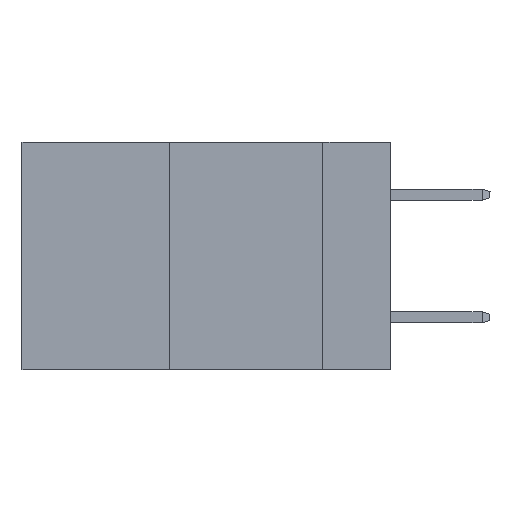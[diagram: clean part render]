
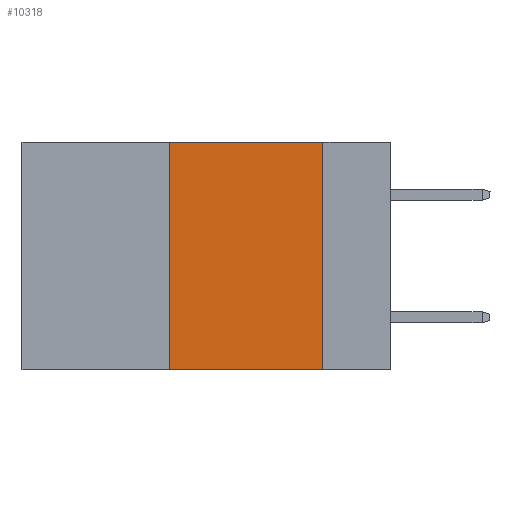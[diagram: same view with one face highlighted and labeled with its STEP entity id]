
A CAD part, left-side view. The second image highlights one B-rep face of the part: STEP entity #10318.
In plain terms, the highlighted planar face has unit normal (-1, 0, 0).
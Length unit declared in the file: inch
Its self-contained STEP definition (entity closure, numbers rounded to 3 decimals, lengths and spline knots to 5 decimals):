
#427 = CARTESIAN_POINT ( 'NONE',  ( 0., 0.11, 0. ) ) ;
#513 = CARTESIAN_POINT ( 'NONE',  ( 0., 0.36, 0. ) ) ;
#746 = EDGE_CURVE ( 'NONE', #7738, #28120, #8736, .T. ) ;
#1292 = VECTOR ( 'NONE', #10631, 39.37008 ) ;
#2387 = LINE ( 'NONE', #29016, #27207 ) ;
#4944 = VECTOR ( 'NONE', #24610, 39.37008 ) ;
#5019 = DIRECTION ( 'NONE',  ( 0., 0., -1. ) ) ;
#6196 = PLANE ( 'NONE',  #29445 ) ;
#7738 = VERTEX_POINT ( 'NONE', #27788 ) ;
#8736 = LINE ( 'NONE', #27074, #4944 ) ;
#10318 = ADVANCED_FACE ( 'NONE', ( #19518 ), #6196, .F. ) ;
#10631 = DIRECTION ( 'NONE',  ( 0., 0., 1. ) ) ;
#11008 = CARTESIAN_POINT ( 'NONE',  ( 0., 0.6, 0. ) ) ;
#14461 = ORIENTED_EDGE ( 'NONE', *, *, #14971, .F. ) ;
#14971 = EDGE_CURVE ( 'NONE', #23796, #28120, #2387, .T. ) ;
#18258 = DIRECTION ( 'NONE',  ( 0., 0., -1. ) ) ;
#19518 = FACE_OUTER_BOUND ( 'NONE', #21424, .T. ) ;
#20540 = ORIENTED_EDGE ( 'NONE', *, *, #25061, .F. ) ;
#20684 = CARTESIAN_POINT ( 'NONE',  ( 0., 0.36, 0. ) ) ;
#21006 = ORIENTED_EDGE ( 'NONE', *, *, #746, .T. ) ;
#21424 = EDGE_LOOP ( 'NONE', ( #14461, #29917, #20540, #21006 ) ) ;
#21808 = VECTOR ( 'NONE', #30907, 39.37008 ) ;
#22946 = CARTESIAN_POINT ( 'NONE',  ( 0., 0.11, -0.37 ) ) ;
#23267 = DIRECTION ( 'NONE',  ( 1., 0., 0. ) ) ;
#23796 = VERTEX_POINT ( 'NONE', #427 ) ;
#24610 = DIRECTION ( 'NONE',  ( 0., -1., 0. ) ) ;
#25061 = EDGE_CURVE ( 'NONE', #7738, #27080, #30635, .T. ) ;
#27074 = CARTESIAN_POINT ( 'NONE',  ( 0., 0.6, -0.37 ) ) ;
#27080 = VERTEX_POINT ( 'NONE', #20684 ) ;
#27207 = VECTOR ( 'NONE', #5019, 39.37008 ) ;
#27525 = LINE ( 'NONE', #28614, #21808 ) ;
#27788 = CARTESIAN_POINT ( 'NONE',  ( 0., 0.36, -0.37 ) ) ;
#28120 = VERTEX_POINT ( 'NONE', #22946 ) ;
#28614 = CARTESIAN_POINT ( 'NONE',  ( 0., 0.6, 0. ) ) ;
#28946 = EDGE_CURVE ( 'NONE', #27080, #23796, #27525, .T. ) ;
#29016 = CARTESIAN_POINT ( 'NONE',  ( 0., 0.11, 0. ) ) ;
#29445 = AXIS2_PLACEMENT_3D ( 'NONE', #11008, #23267, #18258 ) ;
#29917 = ORIENTED_EDGE ( 'NONE', *, *, #28946, .F. ) ;
#30635 = LINE ( 'NONE', #513, #1292 ) ;
#30907 = DIRECTION ( 'NONE',  ( 0., -1., 0. ) ) ;
